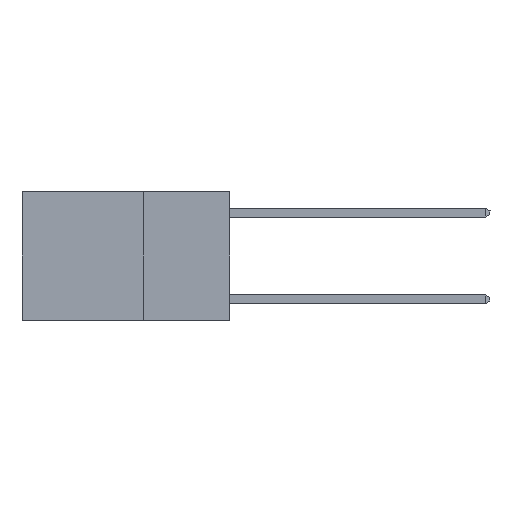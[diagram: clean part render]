
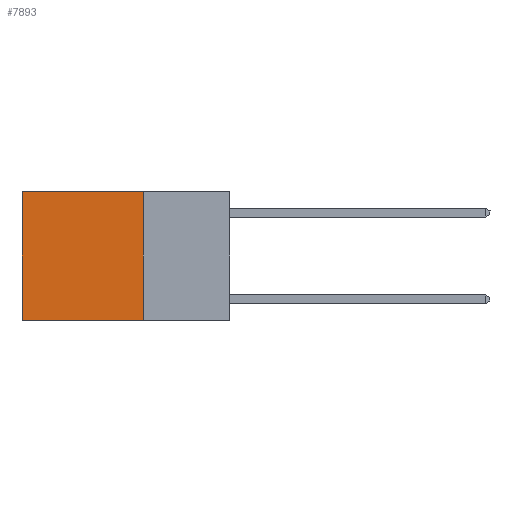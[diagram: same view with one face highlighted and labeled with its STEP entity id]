
A CAD part, left-side view. The second image highlights one B-rep face of the part: STEP entity #7893.
In plain terms, the highlighted planar face has unit normal (-1, 0, 0).
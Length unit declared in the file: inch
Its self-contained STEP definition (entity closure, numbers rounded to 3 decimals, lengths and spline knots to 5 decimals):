
#607 = CARTESIAN_POINT ( 'NONE',  ( 0.2625, 0.25, 0. ) ) ;
#1069 = LINE ( 'NONE', #6794, #1687 ) ;
#1157 = DIRECTION ( 'NONE',  ( 0., 0., -1. ) ) ;
#1272 = EDGE_CURVE ( 'NONE', #2401, #6098, #8415, .T. ) ;
#1687 = VECTOR ( 'NONE', #1157, 39.37008 ) ;
#2401 = VERTEX_POINT ( 'NONE', #17848 ) ;
#2476 = PLANE ( 'NONE',  #6853 ) ;
#2644 = VECTOR ( 'NONE', #6340, 39.37008 ) ;
#3422 = ORIENTED_EDGE ( 'NONE', *, *, #12301, .T. ) ;
#5083 = CARTESIAN_POINT ( 'NONE',  ( 0.2625, 0.25, 0. ) ) ;
#6098 = VERTEX_POINT ( 'NONE', #8132 ) ;
#6340 = DIRECTION ( 'NONE',  ( 0., 1., 0. ) ) ;
#6525 = DIRECTION ( 'NONE',  ( 1., 0., 0. ) ) ;
#6790 = DIRECTION ( 'NONE',  ( 0., 0., -1. ) ) ;
#6794 = CARTESIAN_POINT ( 'NONE',  ( 0.2625, 0.25, 0. ) ) ;
#6826 = CARTESIAN_POINT ( 'NONE',  ( 0.2625, 0.25, -0.37 ) ) ;
#6853 = AXIS2_PLACEMENT_3D ( 'NONE', #8116, #6525, #6790 ) ;
#6914 = EDGE_LOOP ( 'NONE', ( #3422, #17963, #17254, #9928 ) ) ;
#7893 = ADVANCED_FACE ( 'NONE', ( #16929 ), #2476, .F. ) ;
#8116 = CARTESIAN_POINT ( 'NONE',  ( 0.2625, 0.25, 0. ) ) ;
#8132 = CARTESIAN_POINT ( 'NONE',  ( 0.2625, 0.6, -0.37 ) ) ;
#8175 = VECTOR ( 'NONE', #11241, 39.37008 ) ;
#8261 = LINE ( 'NONE', #11273, #10674 ) ;
#8415 = LINE ( 'NONE', #6826, #8175 ) ;
#9928 = ORIENTED_EDGE ( 'NONE', *, *, #16073, .T. ) ;
#10674 = VECTOR ( 'NONE', #13979, 39.37008 ) ;
#10714 = VERTEX_POINT ( 'NONE', #18181 ) ;
#11241 = DIRECTION ( 'NONE',  ( 0., 1., 0. ) ) ;
#11273 = CARTESIAN_POINT ( 'NONE',  ( 0.2625, 0.6, 0. ) ) ;
#11386 = EDGE_CURVE ( 'NONE', #17844, #2401, #1069, .T. ) ;
#12301 = EDGE_CURVE ( 'NONE', #10714, #6098, #8261, .T. ) ;
#13979 = DIRECTION ( 'NONE',  ( 0., 0., -1. ) ) ;
#14879 = LINE ( 'NONE', #607, #2644 ) ;
#16073 = EDGE_CURVE ( 'NONE', #17844, #10714, #14879, .T. ) ;
#16929 = FACE_OUTER_BOUND ( 'NONE', #6914, .T. ) ;
#17254 = ORIENTED_EDGE ( 'NONE', *, *, #11386, .F. ) ;
#17844 = VERTEX_POINT ( 'NONE', #5083 ) ;
#17848 = CARTESIAN_POINT ( 'NONE',  ( 0.2625, 0.25, -0.37 ) ) ;
#17963 = ORIENTED_EDGE ( 'NONE', *, *, #1272, .F. ) ;
#18181 = CARTESIAN_POINT ( 'NONE',  ( 0.2625, 0.6, 0. ) ) ;
